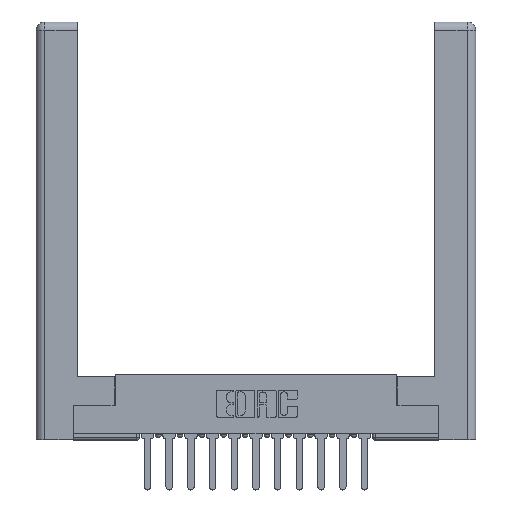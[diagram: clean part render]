
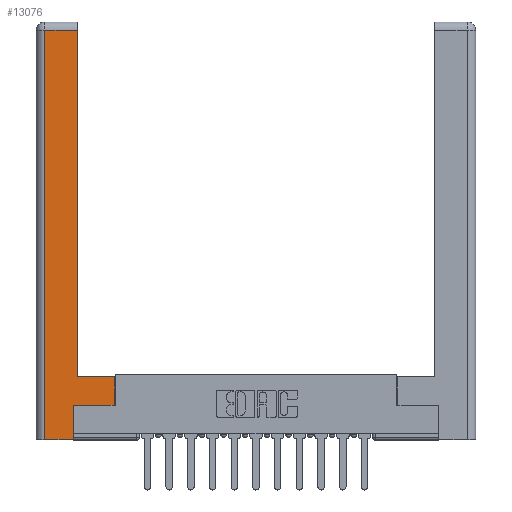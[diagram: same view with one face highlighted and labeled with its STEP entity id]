
A CAD part, top view. The second image highlights one B-rep face of the part: STEP entity #13076.
In plain terms, the highlighted planar face has unit normal (0, 0, 1).
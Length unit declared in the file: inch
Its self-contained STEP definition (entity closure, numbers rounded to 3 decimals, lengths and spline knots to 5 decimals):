
#128 = ORIENTED_EDGE ( 'NONE', *, *, #5787, .T. ) ;
#157 = LINE ( 'NONE', #13790, #15623 ) ;
#793 = VERTEX_POINT ( 'NONE', #1529 ) ;
#828 = PLANE ( 'NONE',  #14475 ) ;
#903 = LINE ( 'NONE', #9606, #7141 ) ;
#1081 = EDGE_LOOP ( 'NONE', ( #12957, #5557, #8242, #15205, #1158, #128, #14873, #13342 ) ) ;
#1158 = ORIENTED_EDGE ( 'NONE', *, *, #12146, .T. ) ;
#1204 = CARTESIAN_POINT ( 'NONE',  ( 0.295, 0.45, 0. ) ) ;
#1404 = CARTESIAN_POINT ( 'NONE',  ( 0.565, 0.245, 0. ) ) ;
#1476 = EDGE_CURVE ( 'NONE', #12639, #10294, #157, .T. ) ;
#1529 = CARTESIAN_POINT ( 'NONE',  ( 0.0615, 0., 0. ) ) ;
#1654 = CARTESIAN_POINT ( 'NONE',  ( 0.265, 0.245, 0. ) ) ;
#2349 = CARTESIAN_POINT ( 'NONE',  ( 0.565, 0.45, 0. ) ) ;
#2587 = DIRECTION ( 'NONE',  ( 1., 0., 0. ) ) ;
#3674 = VECTOR ( 'NONE', #14298, 39.37008 ) ;
#4664 = CARTESIAN_POINT ( 'NONE',  ( 0., 0., 0. ) ) ;
#4984 = DIRECTION ( 'NONE',  ( 0., 1., 0. ) ) ;
#5557 = ORIENTED_EDGE ( 'NONE', *, *, #1476, .T. ) ;
#5787 = EDGE_CURVE ( 'NONE', #14118, #9917, #10584, .T. ) ;
#6850 = CARTESIAN_POINT ( 'NONE',  ( 0.265, 0., 0. ) ) ;
#7141 = VECTOR ( 'NONE', #9366, 39.37008 ) ;
#7208 = FACE_OUTER_BOUND ( 'NONE', #1081, .T. ) ;
#7563 = CARTESIAN_POINT ( 'NONE',  ( 0.565, 0.45, 0. ) ) ;
#7687 = EDGE_CURVE ( 'NONE', #13513, #16158, #9881, .T. ) ;
#7848 = LINE ( 'NONE', #12851, #15761 ) ;
#8242 = ORIENTED_EDGE ( 'NONE', *, *, #14288, .T. ) ;
#8420 = CARTESIAN_POINT ( 'NONE',  ( 0.295, 0.45, 0. ) ) ;
#8459 = DIRECTION ( 'NONE',  ( 0., 0., -1. ) ) ;
#9100 = CARTESIAN_POINT ( 'NONE',  ( 0.0615, 2.94, 0. ) ) ;
#9162 = VECTOR ( 'NONE', #2587, 39.37008 ) ;
#9366 = DIRECTION ( 'NONE',  ( 0., -1., 0. ) ) ;
#9367 = CARTESIAN_POINT ( 'NONE',  ( 0.295, 3., 0. ) ) ;
#9606 = CARTESIAN_POINT ( 'NONE',  ( 0.0615, 0., 0. ) ) ;
#9881 = LINE ( 'NONE', #8420, #12489 ) ;
#9917 = VERTEX_POINT ( 'NONE', #1404 ) ;
#10030 = EDGE_CURVE ( 'NONE', #16158, #12639, #14544, .T. ) ;
#10294 = VERTEX_POINT ( 'NONE', #9100 ) ;
#10584 = LINE ( 'NONE', #12044, #13072 ) ;
#11121 = DIRECTION ( 'NONE',  ( -1., 0., 0. ) ) ;
#11214 = EDGE_CURVE ( 'NONE', #793, #12597, #12500, .T. ) ;
#11608 = EDGE_CURVE ( 'NONE', #9917, #13513, #12325, .T. ) ;
#12044 = CARTESIAN_POINT ( 'NONE',  ( 0.565, 0.245, 0. ) ) ;
#12146 = EDGE_CURVE ( 'NONE', #12597, #14118, #7848, .T. ) ;
#12325 = LINE ( 'NONE', #7563, #14159 ) ;
#12407 = DIRECTION ( 'NONE',  ( 0., 1., 0. ) ) ;
#12489 = VECTOR ( 'NONE', #11121, 39.37008 ) ;
#12500 = LINE ( 'NONE', #13996, #9162 ) ;
#12597 = VERTEX_POINT ( 'NONE', #6850 ) ;
#12639 = VERTEX_POINT ( 'NONE', #14402 ) ;
#12714 = DIRECTION ( 'NONE',  ( -1., 0., 0. ) ) ;
#12851 = CARTESIAN_POINT ( 'NONE',  ( 0.265, 0.245, 0. ) ) ;
#12957 = ORIENTED_EDGE ( 'NONE', *, *, #10030, .T. ) ;
#13072 = VECTOR ( 'NONE', #15682, 39.37008 ) ;
#13076 = ADVANCED_FACE ( 'NONE', ( #7208 ), #828, .F. ) ;
#13342 = ORIENTED_EDGE ( 'NONE', *, *, #7687, .T. ) ;
#13513 = VERTEX_POINT ( 'NONE', #2349 ) ;
#13524 = DIRECTION ( 'NONE',  ( -1., 0., 0. ) ) ;
#13790 = CARTESIAN_POINT ( 'NONE',  ( 0.0615, 2.94, 0. ) ) ;
#13996 = CARTESIAN_POINT ( 'NONE',  ( 0.265, 0., 0. ) ) ;
#14118 = VERTEX_POINT ( 'NONE', #1654 ) ;
#14159 = VECTOR ( 'NONE', #12407, 39.37008 ) ;
#14288 = EDGE_CURVE ( 'NONE', #10294, #793, #903, .T. ) ;
#14298 = DIRECTION ( 'NONE',  ( 0., 1., 0. ) ) ;
#14402 = CARTESIAN_POINT ( 'NONE',  ( 0.295, 2.94, 0. ) ) ;
#14475 = AXIS2_PLACEMENT_3D ( 'NONE', #4664, #8459, #13524 ) ;
#14544 = LINE ( 'NONE', #9367, #3674 ) ;
#14873 = ORIENTED_EDGE ( 'NONE', *, *, #11608, .T. ) ;
#15205 = ORIENTED_EDGE ( 'NONE', *, *, #11214, .T. ) ;
#15623 = VECTOR ( 'NONE', #12714, 39.37008 ) ;
#15682 = DIRECTION ( 'NONE',  ( 1., 0., 0. ) ) ;
#15761 = VECTOR ( 'NONE', #4984, 39.37008 ) ;
#16158 = VERTEX_POINT ( 'NONE', #1204 ) ;
